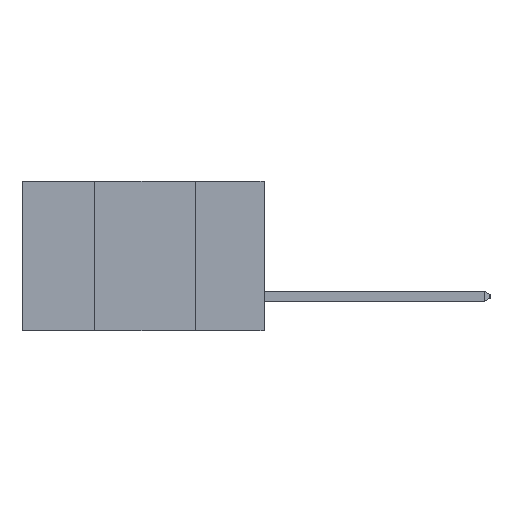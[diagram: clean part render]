
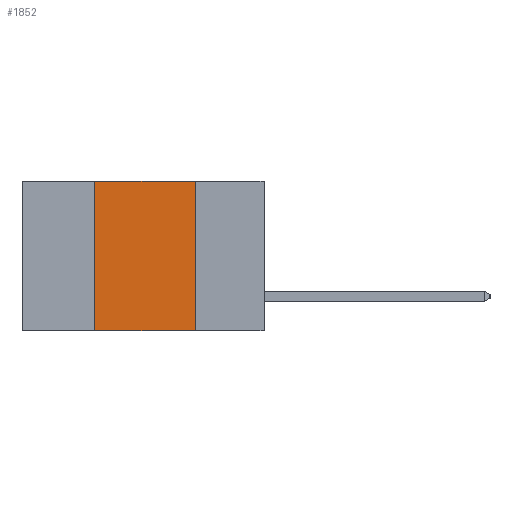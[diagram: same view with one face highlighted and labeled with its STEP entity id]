
A CAD part, left-side view. The second image highlights one B-rep face of the part: STEP entity #1852.
In plain terms, the highlighted planar face has unit normal (-1, 0, 0).
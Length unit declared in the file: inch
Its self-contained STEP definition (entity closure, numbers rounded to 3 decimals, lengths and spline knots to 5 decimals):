
#124 = CARTESIAN_POINT ( 'NONE',  ( 0., 0.6, -0.37 ) ) ;
#323 = EDGE_CURVE ( 'NONE', #9616, #12814, #752, .T. ) ;
#596 = EDGE_LOOP ( 'NONE', ( #7095, #7448, #6276, #5768 ) ) ;
#709 = CARTESIAN_POINT ( 'NONE',  ( 0., 0.42, -0.37 ) ) ;
#752 = LINE ( 'NONE', #124, #4105 ) ;
#1279 = CARTESIAN_POINT ( 'NONE',  ( 0., 0.6, 0. ) ) ;
#1852 = ADVANCED_FACE ( 'NONE', ( #15135 ), #11781, .F. ) ;
#2720 = LINE ( 'NONE', #7781, #9663 ) ;
#3347 = EDGE_CURVE ( 'NONE', #3883, #11248, #16873, .T. ) ;
#3883 = VERTEX_POINT ( 'NONE', #9744 ) ;
#4105 = VECTOR ( 'NONE', #9034, 39.37008 ) ;
#4489 = CARTESIAN_POINT ( 'NONE',  ( 0., 0.6, 0. ) ) ;
#5768 = ORIENTED_EDGE ( 'NONE', *, *, #323, .T. ) ;
#6055 = DIRECTION ( 'NONE',  ( 1., 0., 0. ) ) ;
#6276 = ORIENTED_EDGE ( 'NONE', *, *, #7036, .F. ) ;
#6925 = VECTOR ( 'NONE', #15964, 39.37008 ) ;
#7036 = EDGE_CURVE ( 'NONE', #9616, #3883, #2720, .T. ) ;
#7095 = ORIENTED_EDGE ( 'NONE', *, *, #11205, .F. ) ;
#7448 = ORIENTED_EDGE ( 'NONE', *, *, #3347, .F. ) ;
#7722 = DIRECTION ( 'NONE',  ( 0., 0., 1. ) ) ;
#7781 = CARTESIAN_POINT ( 'NONE',  ( 0., 0.42, -0.37 ) ) ;
#9034 = DIRECTION ( 'NONE',  ( 0., -1., 0. ) ) ;
#9616 = VERTEX_POINT ( 'NONE', #709 ) ;
#9663 = VECTOR ( 'NONE', #7722, 39.37008 ) ;
#9744 = CARTESIAN_POINT ( 'NONE',  ( 0., 0.42, 0. ) ) ;
#10742 = CARTESIAN_POINT ( 'NONE',  ( 0., 0.17, 0. ) ) ;
#11205 = EDGE_CURVE ( 'NONE', #11248, #12814, #17569, .T. ) ;
#11248 = VERTEX_POINT ( 'NONE', #10742 ) ;
#11529 = AXIS2_PLACEMENT_3D ( 'NONE', #1279, #6055, #12904 ) ;
#11781 = PLANE ( 'NONE',  #11529 ) ;
#12814 = VERTEX_POINT ( 'NONE', #15366 ) ;
#12904 = DIRECTION ( 'NONE',  ( 0., 0., -1. ) ) ;
#12983 = VECTOR ( 'NONE', #14134, 39.37008 ) ;
#14134 = DIRECTION ( 'NONE',  ( 0., -1., 0. ) ) ;
#14656 = CARTESIAN_POINT ( 'NONE',  ( 0., 0.17, -0.37 ) ) ;
#15135 = FACE_OUTER_BOUND ( 'NONE', #596, .T. ) ;
#15366 = CARTESIAN_POINT ( 'NONE',  ( 0., 0.17, -0.37 ) ) ;
#15964 = DIRECTION ( 'NONE',  ( 0., 0., -1. ) ) ;
#16873 = LINE ( 'NONE', #4489, #12983 ) ;
#17569 = LINE ( 'NONE', #14656, #6925 ) ;
